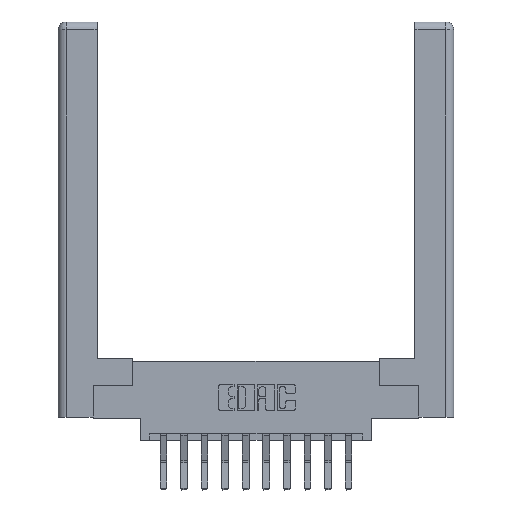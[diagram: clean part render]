
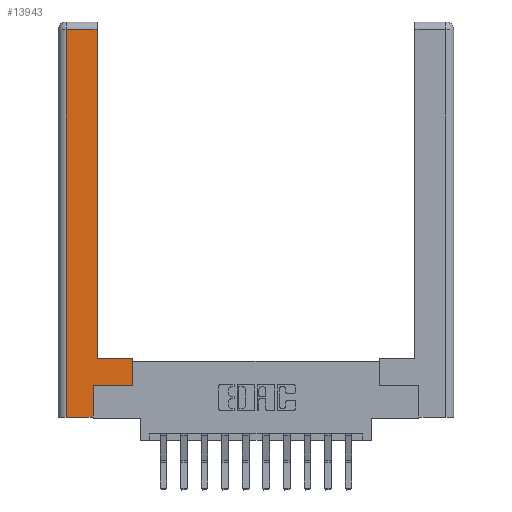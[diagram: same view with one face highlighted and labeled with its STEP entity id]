
A CAD part, top view. The second image highlights one B-rep face of the part: STEP entity #13943.
In plain terms, the highlighted planar face has unit normal (0, 0, 1).
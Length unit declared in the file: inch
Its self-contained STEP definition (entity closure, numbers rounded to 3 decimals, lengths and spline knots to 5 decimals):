
#9 = CARTESIAN_POINT ( 'NONE',  ( 0.565, 0.45, 0. ) ) ;
#195 = DIRECTION ( 'NONE',  ( -1., 0., 0. ) ) ;
#658 = EDGE_CURVE ( 'NONE', #9006, #13932, #10241, .T. ) ;
#675 = ORIENTED_EDGE ( 'NONE', *, *, #658, .T. ) ;
#702 = LINE ( 'NONE', #5835, #6446 ) ;
#873 = VERTEX_POINT ( 'NONE', #1915 ) ;
#1005 = CARTESIAN_POINT ( 'NONE',  ( 0., 0., 0. ) ) ;
#1106 = CARTESIAN_POINT ( 'NONE',  ( 0.265, 0.245, 0. ) ) ;
#1484 = VECTOR ( 'NONE', #6077, 39.37008 ) ;
#1650 = CARTESIAN_POINT ( 'NONE',  ( 0.295, 2.94, 0. ) ) ;
#1689 = EDGE_CURVE ( 'NONE', #4210, #4844, #1835, .T. ) ;
#1835 = LINE ( 'NONE', #6939, #5425 ) ;
#1915 = CARTESIAN_POINT ( 'NONE',  ( 0.565, 0.245, 0. ) ) ;
#2153 = DIRECTION ( 'NONE',  ( -1., 0., 0. ) ) ;
#2459 = ORIENTED_EDGE ( 'NONE', *, *, #8556, .T. ) ;
#2721 = CARTESIAN_POINT ( 'NONE',  ( 0.265, 0., 0. ) ) ;
#3112 = LINE ( 'NONE', #10240, #11832 ) ;
#3444 = VECTOR ( 'NONE', #7086, 39.37008 ) ;
#3534 = VECTOR ( 'NONE', #12399, 39.37008 ) ;
#3668 = AXIS2_PLACEMENT_3D ( 'NONE', #1005, #9000, #2153 ) ;
#4210 = VERTEX_POINT ( 'NONE', #1650 ) ;
#4463 = ORIENTED_EDGE ( 'NONE', *, *, #10587, .T. ) ;
#4570 = DIRECTION ( 'NONE',  ( 0., 1., 0. ) ) ;
#4721 = ORIENTED_EDGE ( 'NONE', *, *, #12326, .T. ) ;
#4730 = CARTESIAN_POINT ( 'NONE',  ( 0.295, 3., 0. ) ) ;
#4746 = CARTESIAN_POINT ( 'NONE',  ( 0.295, 0.45, 0. ) ) ;
#4844 = VERTEX_POINT ( 'NONE', #7402 ) ;
#5425 = VECTOR ( 'NONE', #195, 39.37008 ) ;
#5800 = ORIENTED_EDGE ( 'NONE', *, *, #8784, .T. ) ;
#5835 = CARTESIAN_POINT ( 'NONE',  ( 0.265, 0.245, 0. ) ) ;
#6077 = DIRECTION ( 'NONE',  ( 1., 0., 0. ) ) ;
#6338 = EDGE_CURVE ( 'NONE', #13932, #8742, #702, .T. ) ;
#6376 = CARTESIAN_POINT ( 'NONE',  ( 0.565, 0.45, 0. ) ) ;
#6446 = VECTOR ( 'NONE', #13786, 39.37008 ) ;
#6773 = DIRECTION ( 'NONE',  ( 1., 0., 0. ) ) ;
#6811 = CARTESIAN_POINT ( 'NONE',  ( 0.265, 0., 0. ) ) ;
#6939 = CARTESIAN_POINT ( 'NONE',  ( 0.0615, 2.94, 0. ) ) ;
#6985 = CARTESIAN_POINT ( 'NONE',  ( 0.0615, 0., 0. ) ) ;
#7086 = DIRECTION ( 'NONE',  ( 0., -1., 0. ) ) ;
#7293 = EDGE_LOOP ( 'NONE', ( #4463, #8743, #4721, #675, #8646, #11035, #5800, #2459 ) ) ;
#7402 = CARTESIAN_POINT ( 'NONE',  ( 0.0615, 2.94, 0. ) ) ;
#7492 = VECTOR ( 'NONE', #4570, 39.37008 ) ;
#8556 = EDGE_CURVE ( 'NONE', #12233, #9101, #11028, .T. ) ;
#8646 = ORIENTED_EDGE ( 'NONE', *, *, #6338, .T. ) ;
#8742 = VERTEX_POINT ( 'NONE', #1106 ) ;
#8743 = ORIENTED_EDGE ( 'NONE', *, *, #1689, .T. ) ;
#8784 = EDGE_CURVE ( 'NONE', #873, #12233, #14078, .T. ) ;
#9000 = DIRECTION ( 'NONE',  ( 0., 0., -1. ) ) ;
#9006 = VERTEX_POINT ( 'NONE', #11512 ) ;
#9101 = VERTEX_POINT ( 'NONE', #4746 ) ;
#9581 = LINE ( 'NONE', #4730, #13312 ) ;
#10240 = CARTESIAN_POINT ( 'NONE',  ( 0.565, 0.245, 0. ) ) ;
#10241 = LINE ( 'NONE', #2721, #1484 ) ;
#10242 = DIRECTION ( 'NONE',  ( 0., 1., 0. ) ) ;
#10587 = EDGE_CURVE ( 'NONE', #9101, #4210, #9581, .T. ) ;
#11028 = LINE ( 'NONE', #11335, #3534 ) ;
#11035 = ORIENTED_EDGE ( 'NONE', *, *, #12144, .T. ) ;
#11335 = CARTESIAN_POINT ( 'NONE',  ( 0.295, 0.45, 0. ) ) ;
#11512 = CARTESIAN_POINT ( 'NONE',  ( 0.0615, 0., 0. ) ) ;
#11660 = LINE ( 'NONE', #6985, #3444 ) ;
#11832 = VECTOR ( 'NONE', #6773, 39.37008 ) ;
#12144 = EDGE_CURVE ( 'NONE', #8742, #873, #3112, .T. ) ;
#12233 = VERTEX_POINT ( 'NONE', #6376 ) ;
#12326 = EDGE_CURVE ( 'NONE', #4844, #9006, #11660, .T. ) ;
#12399 = DIRECTION ( 'NONE',  ( -1., 0., 0. ) ) ;
#12642 = FACE_OUTER_BOUND ( 'NONE', #7293, .T. ) ;
#13312 = VECTOR ( 'NONE', #10242, 39.37008 ) ;
#13786 = DIRECTION ( 'NONE',  ( 0., 1., 0. ) ) ;
#13932 = VERTEX_POINT ( 'NONE', #6811 ) ;
#13943 = ADVANCED_FACE ( 'NONE', ( #12642 ), #14656, .F. ) ;
#14078 = LINE ( 'NONE', #9, #7492 ) ;
#14656 = PLANE ( 'NONE',  #3668 ) ;
